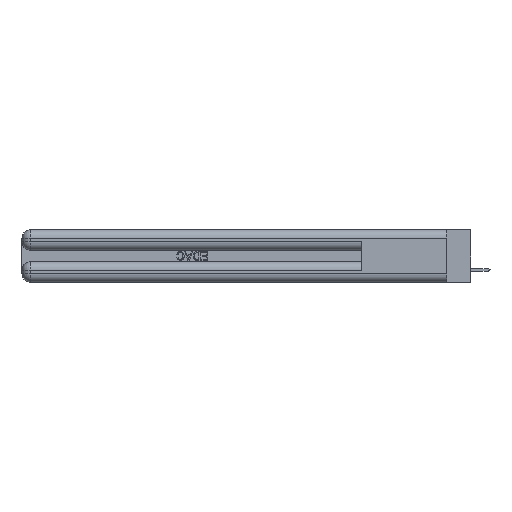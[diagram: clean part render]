
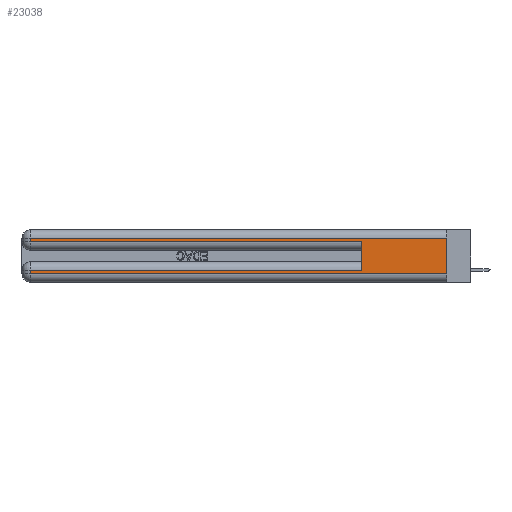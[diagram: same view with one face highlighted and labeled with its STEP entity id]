
A CAD part, left-side view. The second image highlights one B-rep face of the part: STEP entity #23038.
In plain terms, the highlighted planar face has unit normal (-1, 0, 0).
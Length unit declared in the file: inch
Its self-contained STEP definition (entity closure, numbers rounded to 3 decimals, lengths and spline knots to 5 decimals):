
#307 = CARTESIAN_POINT ( 'NONE',  ( 0., 0., 0.06 ) ) ;
#399 = CARTESIAN_POINT ( 'NONE',  ( 0., 0., 0.31 ) ) ;
#1252 = LINE ( 'NONE', #26611, #35849 ) ;
#2280 = DIRECTION ( 'NONE',  ( 1., 0., 0. ) ) ;
#3352 = VECTOR ( 'NONE', #31851, 39.37008 ) ;
#3519 = DIRECTION ( 'NONE',  ( 0., -1., 0. ) ) ;
#3622 = CARTESIAN_POINT ( 'NONE',  ( 0., 0., 0.06 ) ) ;
#3791 = CARTESIAN_POINT ( 'NONE',  ( 0., 2.94, 0.085 ) ) ;
#4635 = VERTEX_POINT ( 'NONE', #24848 ) ;
#4713 = CARTESIAN_POINT ( 'NONE',  ( 0., 0.6, 0.285 ) ) ;
#5275 = EDGE_LOOP ( 'NONE', ( #6871, #30107, #26149, #18878, #9043, #13986, #32095, #6601 ) ) ;
#5597 = AXIS2_PLACEMENT_3D ( 'NONE', #30714, #2280, #21632 ) ;
#6011 = EDGE_CURVE ( 'NONE', #11513, #39917, #39273, .T. ) ;
#6601 = ORIENTED_EDGE ( 'NONE', *, *, #39179, .T. ) ;
#6871 = ORIENTED_EDGE ( 'NONE', *, *, #21488, .F. ) ;
#7555 = EDGE_CURVE ( 'NONE', #8986, #4635, #30652, .T. ) ;
#8986 = VERTEX_POINT ( 'NONE', #9869 ) ;
#8994 = VECTOR ( 'NONE', #24299, 39.37008 ) ;
#9043 = ORIENTED_EDGE ( 'NONE', *, *, #21935, .F. ) ;
#9592 = VERTEX_POINT ( 'NONE', #307 ) ;
#9869 = CARTESIAN_POINT ( 'NONE',  ( 0., 2.94, 0.31 ) ) ;
#11309 = DIRECTION ( 'NONE',  ( 0., 1., 0. ) ) ;
#11513 = VERTEX_POINT ( 'NONE', #3791 ) ;
#12302 = CARTESIAN_POINT ( 'NONE',  ( 0., 2.94, 0.37 ) ) ;
#13586 = EDGE_CURVE ( 'NONE', #4635, #24468, #26752, .T. ) ;
#13986 = ORIENTED_EDGE ( 'NONE', *, *, #38360, .T. ) ;
#14460 = CARTESIAN_POINT ( 'NONE',  ( 0., 2.94, 0.06 ) ) ;
#15139 = VECTOR ( 'NONE', #11309, 39.37008 ) ;
#15349 = DIRECTION ( 'NONE',  ( 0., 0., -1. ) ) ;
#17401 = CARTESIAN_POINT ( 'NONE',  ( 0., 2.94, 0.37 ) ) ;
#18848 = CARTESIAN_POINT ( 'NONE',  ( 0., 0., 0.37 ) ) ;
#18878 = ORIENTED_EDGE ( 'NONE', *, *, #13586, .T. ) ;
#19269 = LINE ( 'NONE', #3622, #3352 ) ;
#19300 = VECTOR ( 'NONE', #15349, 39.37008 ) ;
#20391 = DIRECTION ( 'NONE',  ( 0., 0., 1. ) ) ;
#21488 = EDGE_CURVE ( 'NONE', #23626, #9592, #40321, .T. ) ;
#21632 = DIRECTION ( 'NONE',  ( 0., 0., -1. ) ) ;
#21935 = EDGE_CURVE ( 'NONE', #33948, #24468, #1252, .T. ) ;
#23038 = ADVANCED_FACE ( 'NONE', ( #33817 ), #30295, .F. ) ;
#23626 = VERTEX_POINT ( 'NONE', #399 ) ;
#24299 = DIRECTION ( 'NONE',  ( 0., 1., 0. ) ) ;
#24468 = VERTEX_POINT ( 'NONE', #4713 ) ;
#24848 = CARTESIAN_POINT ( 'NONE',  ( 0., 2.94, 0.285 ) ) ;
#26149 = ORIENTED_EDGE ( 'NONE', *, *, #7555, .T. ) ;
#26580 = LINE ( 'NONE', #39575, #15139 ) ;
#26611 = CARTESIAN_POINT ( 'NONE',  ( 0., 0.6, 0.145 ) ) ;
#26673 = EDGE_CURVE ( 'NONE', #23626, #8986, #28005, .T. ) ;
#26752 = LINE ( 'NONE', #31756, #33217 ) ;
#28005 = LINE ( 'NONE', #36890, #8994 ) ;
#28859 = CARTESIAN_POINT ( 'NONE',  ( 0., 0.6, 0.085 ) ) ;
#30107 = ORIENTED_EDGE ( 'NONE', *, *, #26673, .T. ) ;
#30295 = PLANE ( 'NONE',  #5597 ) ;
#30652 = LINE ( 'NONE', #12302, #37623 ) ;
#30714 = CARTESIAN_POINT ( 'NONE',  ( 0., 0., 0.37 ) ) ;
#31756 = CARTESIAN_POINT ( 'NONE',  ( 0., 0., 0.285 ) ) ;
#31851 = DIRECTION ( 'NONE',  ( 0., -1., 0. ) ) ;
#32095 = ORIENTED_EDGE ( 'NONE', *, *, #6011, .T. ) ;
#33217 = VECTOR ( 'NONE', #3519, 39.37008 ) ;
#33817 = FACE_OUTER_BOUND ( 'NONE', #5275, .T. ) ;
#33948 = VERTEX_POINT ( 'NONE', #28859 ) ;
#35849 = VECTOR ( 'NONE', #20391, 39.37008 ) ;
#36596 = DIRECTION ( 'NONE',  ( 0., 0., -1. ) ) ;
#36890 = CARTESIAN_POINT ( 'NONE',  ( 0., 0., 0.31 ) ) ;
#37623 = VECTOR ( 'NONE', #40565, 39.37008 ) ;
#38199 = VECTOR ( 'NONE', #36596, 39.37008 ) ;
#38360 = EDGE_CURVE ( 'NONE', #33948, #11513, #26580, .T. ) ;
#39179 = EDGE_CURVE ( 'NONE', #39917, #9592, #19269, .T. ) ;
#39273 = LINE ( 'NONE', #17401, #38199 ) ;
#39575 = CARTESIAN_POINT ( 'NONE',  ( 0., 0., 0.085 ) ) ;
#39917 = VERTEX_POINT ( 'NONE', #14460 ) ;
#40321 = LINE ( 'NONE', #18848, #19300 ) ;
#40565 = DIRECTION ( 'NONE',  ( 0., 0., -1. ) ) ;
